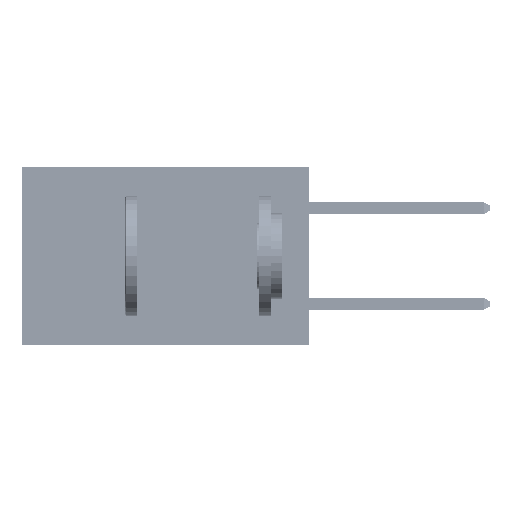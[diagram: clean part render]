
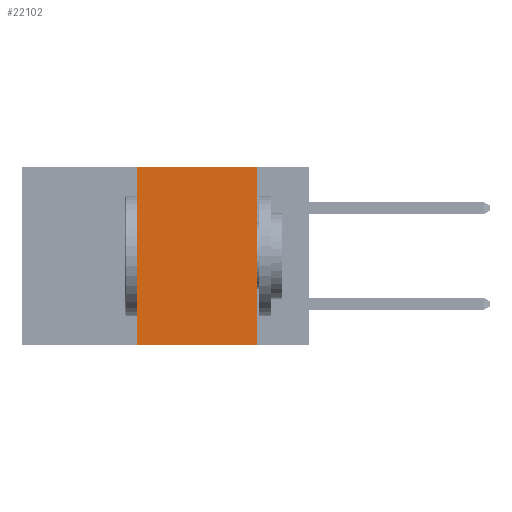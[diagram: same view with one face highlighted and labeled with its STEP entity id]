
A CAD part, left-side view. The second image highlights one B-rep face of the part: STEP entity #22102.
In plain terms, the highlighted planar face has unit normal (-1, 0, 0).
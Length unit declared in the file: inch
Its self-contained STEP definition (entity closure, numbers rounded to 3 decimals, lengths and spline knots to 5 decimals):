
#3025 = CARTESIAN_POINT ( 'NONE',  ( 0., 0.11, 0. ) ) ;
#3401 = VECTOR ( 'NONE', #3845, 39.37008 ) ;
#3458 = DIRECTION ( 'NONE',  ( 0., 0., -1. ) ) ;
#3568 = VECTOR ( 'NONE', #30585, 39.37008 ) ;
#3845 = DIRECTION ( 'NONE',  ( 0., 0., 1. ) ) ;
#4252 = CARTESIAN_POINT ( 'NONE',  ( 0., 0.36, -0.37 ) ) ;
#7544 = LINE ( 'NONE', #3025, #34212 ) ;
#10432 = CARTESIAN_POINT ( 'NONE',  ( 0., 0.6, 0. ) ) ;
#12527 = ORIENTED_EDGE ( 'NONE', *, *, #38518, .F. ) ;
#12857 = VERTEX_POINT ( 'NONE', #13889 ) ;
#13555 = FACE_OUTER_BOUND ( 'NONE', #37032, .T. ) ;
#13889 = CARTESIAN_POINT ( 'NONE',  ( 0., 0.11, 0. ) ) ;
#14067 = CARTESIAN_POINT ( 'NONE',  ( 0., 0.36, 0. ) ) ;
#19003 = DIRECTION ( 'NONE',  ( 1., 0., 0. ) ) ;
#19650 = EDGE_CURVE ( 'NONE', #12857, #29445, #7544, .T. ) ;
#21191 = VERTEX_POINT ( 'NONE', #14067 ) ;
#21957 = CARTESIAN_POINT ( 'NONE',  ( 0., 0.11, -0.37 ) ) ;
#22102 = ADVANCED_FACE ( 'NONE', ( #13555 ), #47134, .F. ) ;
#23464 = CARTESIAN_POINT ( 'NONE',  ( 0., 0.6, -0.37 ) ) ;
#24855 = EDGE_CURVE ( 'NONE', #43923, #29445, #43674, .T. ) ;
#28232 = LINE ( 'NONE', #36099, #3401 ) ;
#29010 = AXIS2_PLACEMENT_3D ( 'NONE', #50947, #19003, #3458 ) ;
#29445 = VERTEX_POINT ( 'NONE', #21957 ) ;
#29642 = LINE ( 'NONE', #10432, #3568 ) ;
#30585 = DIRECTION ( 'NONE',  ( 0., -1., 0. ) ) ;
#30767 = DIRECTION ( 'NONE',  ( 0., 0., -1. ) ) ;
#32465 = EDGE_CURVE ( 'NONE', #43923, #21191, #28232, .T. ) ;
#34212 = VECTOR ( 'NONE', #30767, 39.37008 ) ;
#34392 = ORIENTED_EDGE ( 'NONE', *, *, #24855, .T. ) ;
#35962 = ORIENTED_EDGE ( 'NONE', *, *, #32465, .F. ) ;
#36099 = CARTESIAN_POINT ( 'NONE',  ( 0., 0.36, 0. ) ) ;
#37032 = EDGE_LOOP ( 'NONE', ( #38156, #12527, #35962, #34392 ) ) ;
#38156 = ORIENTED_EDGE ( 'NONE', *, *, #19650, .F. ) ;
#38518 = EDGE_CURVE ( 'NONE', #21191, #12857, #29642, .T. ) ;
#39483 = DIRECTION ( 'NONE',  ( 0., -1., 0. ) ) ;
#43674 = LINE ( 'NONE', #23464, #45491 ) ;
#43923 = VERTEX_POINT ( 'NONE', #4252 ) ;
#45491 = VECTOR ( 'NONE', #39483, 39.37008 ) ;
#47134 = PLANE ( 'NONE',  #29010 ) ;
#50947 = CARTESIAN_POINT ( 'NONE',  ( 0., 0.6, 0. ) ) ;
